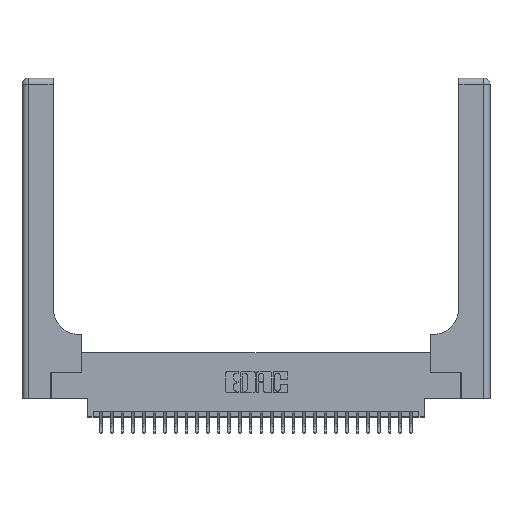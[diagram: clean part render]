
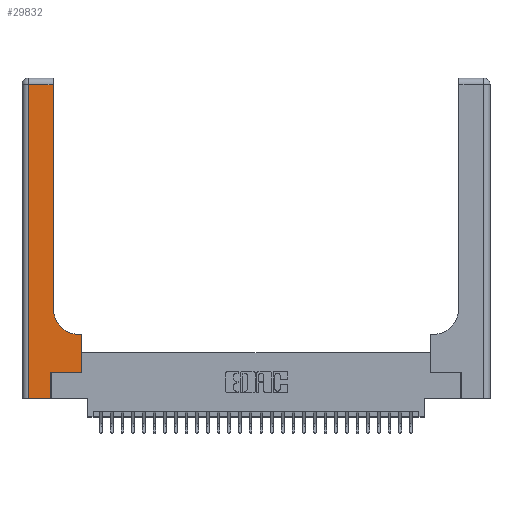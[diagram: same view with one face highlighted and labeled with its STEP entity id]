
A CAD part, top view. The second image highlights one B-rep face of the part: STEP entity #29832.
In plain terms, the highlighted planar face has unit normal (0, 0, 1).
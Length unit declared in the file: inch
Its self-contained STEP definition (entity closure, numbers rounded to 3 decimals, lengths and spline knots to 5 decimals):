
#233 = CARTESIAN_POINT ( 'NONE',  ( 0., 2.94, 0.37 ) ) ;
#547 = CARTESIAN_POINT ( 'NONE',  ( 0.2915, 0.85, 0.37 ) ) ;
#561 = VECTOR ( 'NONE', #9769, 39.37008 ) ;
#562 = CARTESIAN_POINT ( 'NONE',  ( 0.269, 0., 0.37 ) ) ;
#1122 = ORIENTED_EDGE ( 'NONE', *, *, #10202, .T. ) ;
#1525 = DIRECTION ( 'NONE',  ( 0., 0., -1. ) ) ;
#1700 = CARTESIAN_POINT ( 'NONE',  ( 0.06, 3., 0.37 ) ) ;
#1803 = AXIS2_PLACEMENT_3D ( 'NONE', #29950, #1525, #18269 ) ;
#1871 = VECTOR ( 'NONE', #4103, 39.37008 ) ;
#1876 = ORIENTED_EDGE ( 'NONE', *, *, #2589, .T. ) ;
#2311 = EDGE_CURVE ( 'NONE', #14298, #29334, #2448, .T. ) ;
#2448 = LINE ( 'NONE', #27274, #20792 ) ;
#2589 = EDGE_CURVE ( 'NONE', #25557, #3497, #25897, .T. ) ;
#3497 = VERTEX_POINT ( 'NONE', #11024 ) ;
#3557 = VERTEX_POINT ( 'NONE', #30141 ) ;
#3619 = EDGE_CURVE ( 'NONE', #26056, #14298, #16239, .T. ) ;
#3638 = DIRECTION ( 'NONE',  ( 0., 1., 0. ) ) ;
#4103 = DIRECTION ( 'NONE',  ( 0., -1., 0. ) ) ;
#5386 = VECTOR ( 'NONE', #11931, 39.37008 ) ;
#5613 = LINE ( 'NONE', #29679, #29338 ) ;
#5773 = CARTESIAN_POINT ( 'NONE',  ( 0., 0., 0.37 ) ) ;
#5954 = CARTESIAN_POINT ( 'NONE',  ( 0.2915, 2.94, 0.37 ) ) ;
#6264 = VECTOR ( 'NONE', #18515, 39.37008 ) ;
#6793 = CARTESIAN_POINT ( 'NONE',  ( 0.5415, 0.85, 0.37 ) ) ;
#7224 = AXIS2_PLACEMENT_3D ( 'NONE', #6793, #23494, #9225 ) ;
#7412 = VERTEX_POINT ( 'NONE', #562 ) ;
#9225 = DIRECTION ( 'NONE',  ( 1., 0., 0. ) ) ;
#9769 = DIRECTION ( 'NONE',  ( -1., 0., 0. ) ) ;
#10202 = EDGE_CURVE ( 'NONE', #27437, #25557, #5613, .T. ) ;
#11024 = CARTESIAN_POINT ( 'NONE',  ( 0.06, 2.94, 0.37 ) ) ;
#11442 = CARTESIAN_POINT ( 'NONE',  ( 0.5585, 0.25, 0.37 ) ) ;
#11746 = LINE ( 'NONE', #21369, #5386 ) ;
#11931 = DIRECTION ( 'NONE',  ( 1., 0., 0. ) ) ;
#14236 = LINE ( 'NONE', #5773, #26116 ) ;
#14298 = VERTEX_POINT ( 'NONE', #18207 ) ;
#15963 = CIRCLE ( 'NONE', #7224, 0.25 ) ;
#16239 = LINE ( 'NONE', #11442, #21878 ) ;
#17847 = FACE_OUTER_BOUND ( 'NONE', #20204, .T. ) ;
#17912 = EDGE_CURVE ( 'NONE', #25258, #26056, #11746, .T. ) ;
#18207 = CARTESIAN_POINT ( 'NONE',  ( 0.5585, 0.6, 0.37 ) ) ;
#18269 = DIRECTION ( 'NONE',  ( -1., 0., 0. ) ) ;
#18395 = ORIENTED_EDGE ( 'NONE', *, *, #27086, .T. ) ;
#18515 = DIRECTION ( 'NONE',  ( 0., 1., 0. ) ) ;
#18832 = CARTESIAN_POINT ( 'NONE',  ( 0.269, 0.25, 0.37 ) ) ;
#19695 = ORIENTED_EDGE ( 'NONE', *, *, #29560, .T. ) ;
#20204 = EDGE_LOOP ( 'NONE', ( #1122, #1876, #18395, #28556, #19695, #27790, #23534, #29180, #24880 ) ) ;
#20792 = VECTOR ( 'NONE', #22698, 39.37008 ) ;
#20983 = LINE ( 'NONE', #1700, #1871 ) ;
#21369 = CARTESIAN_POINT ( 'NONE',  ( 0.269, 0.25, 0.37 ) ) ;
#21878 = VECTOR ( 'NONE', #23341, 39.37008 ) ;
#22698 = DIRECTION ( 'NONE',  ( -1., 0., 0. ) ) ;
#23341 = DIRECTION ( 'NONE',  ( 0., 1., 0. ) ) ;
#23494 = DIRECTION ( 'NONE',  ( 0., 0., -1. ) ) ;
#23534 = ORIENTED_EDGE ( 'NONE', *, *, #3619, .T. ) ;
#24845 = DIRECTION ( 'NONE',  ( 1., 0., 0. ) ) ;
#24880 = ORIENTED_EDGE ( 'NONE', *, *, #29613, .T. ) ;
#25258 = VERTEX_POINT ( 'NONE', #18832 ) ;
#25557 = VERTEX_POINT ( 'NONE', #5954 ) ;
#25897 = LINE ( 'NONE', #233, #561 ) ;
#26056 = VERTEX_POINT ( 'NONE', #28941 ) ;
#26116 = VECTOR ( 'NONE', #24845, 39.37008 ) ;
#26877 = EDGE_CURVE ( 'NONE', #3557, #7412, #14236, .T. ) ;
#27086 = EDGE_CURVE ( 'NONE', #3497, #3557, #20983, .T. ) ;
#27274 = CARTESIAN_POINT ( 'NONE',  ( 0.2915, 0.6, 0.37 ) ) ;
#27437 = VERTEX_POINT ( 'NONE', #547 ) ;
#27628 = PLANE ( 'NONE',  #1803 ) ;
#27790 = ORIENTED_EDGE ( 'NONE', *, *, #17912, .T. ) ;
#28556 = ORIENTED_EDGE ( 'NONE', *, *, #26877, .T. ) ;
#28941 = CARTESIAN_POINT ( 'NONE',  ( 0.5585, 0.25, 0.37 ) ) ;
#29180 = ORIENTED_EDGE ( 'NONE', *, *, #2311, .T. ) ;
#29284 = CARTESIAN_POINT ( 'NONE',  ( 0.5415, 0.6, 0.37 ) ) ;
#29334 = VERTEX_POINT ( 'NONE', #29284 ) ;
#29338 = VECTOR ( 'NONE', #3638, 39.37008 ) ;
#29560 = EDGE_CURVE ( 'NONE', #7412, #25258, #29978, .T. ) ;
#29613 = EDGE_CURVE ( 'NONE', #29334, #27437, #15963, .T. ) ;
#29679 = CARTESIAN_POINT ( 'NONE',  ( 0.2915, 3., 0.37 ) ) ;
#29832 = ADVANCED_FACE ( 'NONE', ( #17847 ), #27628, .F. ) ;
#29950 = CARTESIAN_POINT ( 'NONE',  ( 0., 3., 0.37 ) ) ;
#29978 = LINE ( 'NONE', #30193, #6264 ) ;
#30141 = CARTESIAN_POINT ( 'NONE',  ( 0.06, 0., 0.37 ) ) ;
#30193 = CARTESIAN_POINT ( 'NONE',  ( 0.269, 0., 0.37 ) ) ;
